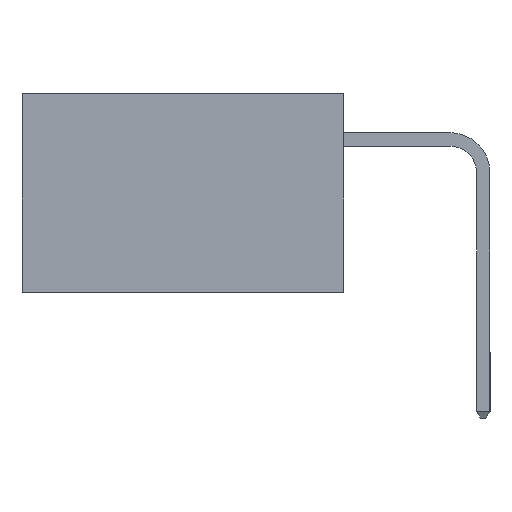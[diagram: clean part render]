
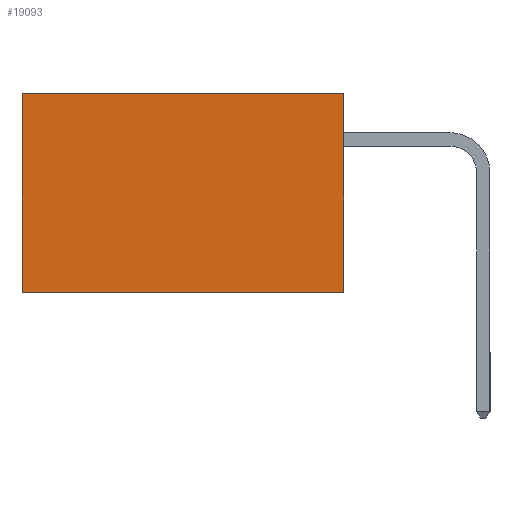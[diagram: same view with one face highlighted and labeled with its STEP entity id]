
A CAD part, left-side view. The second image highlights one B-rep face of the part: STEP entity #19093.
In plain terms, the highlighted planar face has unit normal (-1, 0, 0).
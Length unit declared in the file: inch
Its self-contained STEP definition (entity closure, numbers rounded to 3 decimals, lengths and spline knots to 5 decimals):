
#627 = DIRECTION ( 'NONE',  ( 0., 0., -1. ) ) ;
#920 = LINE ( 'NONE', #1211, #15203 ) ;
#930 = ORIENTED_EDGE ( 'NONE', *, *, #7329, .T. ) ;
#1211 = CARTESIAN_POINT ( 'NONE',  ( 0.2615, 0., 0. ) ) ;
#2139 = LINE ( 'NONE', #5293, #7869 ) ;
#2337 = CARTESIAN_POINT ( 'NONE',  ( 0.2615, 0., -0.37 ) ) ;
#5293 = CARTESIAN_POINT ( 'NONE',  ( 0.2615, 0.6, -0.37 ) ) ;
#5591 = VECTOR ( 'NONE', #17047, 39.37008 ) ;
#5892 = EDGE_CURVE ( 'NONE', #15554, #14529, #18136, .T. ) ;
#6039 = FACE_OUTER_BOUND ( 'NONE', #9363, .T. ) ;
#6125 = VERTEX_POINT ( 'NONE', #16425 ) ;
#7064 = VECTOR ( 'NONE', #15613, 39.37008 ) ;
#7329 = EDGE_CURVE ( 'NONE', #15351, #14529, #2139, .T. ) ;
#7866 = DIRECTION ( 'NONE',  ( 0., 0., -1. ) ) ;
#7869 = VECTOR ( 'NONE', #627, 39.37008 ) ;
#9349 = LINE ( 'NONE', #12423, #7064 ) ;
#9363 = EDGE_LOOP ( 'NONE', ( #930, #19481, #10016, #16071 ) ) ;
#9390 = PLANE ( 'NONE',  #11045 ) ;
#10016 = ORIENTED_EDGE ( 'NONE', *, *, #15057, .F. ) ;
#10208 = DIRECTION ( 'NONE',  ( 0., 1., 0. ) ) ;
#11045 = AXIS2_PLACEMENT_3D ( 'NONE', #13699, #15649, #7866 ) ;
#12305 = EDGE_CURVE ( 'NONE', #6125, #15351, #920, .T. ) ;
#12423 = CARTESIAN_POINT ( 'NONE',  ( 0.2615, 0., -0.37 ) ) ;
#13699 = CARTESIAN_POINT ( 'NONE',  ( 0.2615, 0., -0.37 ) ) ;
#14474 = CARTESIAN_POINT ( 'NONE',  ( 0.2615, 0.6, 0. ) ) ;
#14529 = VERTEX_POINT ( 'NONE', #14966 ) ;
#14966 = CARTESIAN_POINT ( 'NONE',  ( 0.2615, 0.6, -0.37 ) ) ;
#15057 = EDGE_CURVE ( 'NONE', #6125, #15554, #9349, .T. ) ;
#15203 = VECTOR ( 'NONE', #10208, 39.37008 ) ;
#15351 = VERTEX_POINT ( 'NONE', #14474 ) ;
#15554 = VERTEX_POINT ( 'NONE', #2337 ) ;
#15613 = DIRECTION ( 'NONE',  ( 0., 0., -1. ) ) ;
#15649 = DIRECTION ( 'NONE',  ( 1., 0., 0. ) ) ;
#16071 = ORIENTED_EDGE ( 'NONE', *, *, #12305, .T. ) ;
#16425 = CARTESIAN_POINT ( 'NONE',  ( 0.2615, 0., 0. ) ) ;
#17047 = DIRECTION ( 'NONE',  ( 0., 1., 0. ) ) ;
#18136 = LINE ( 'NONE', #19695, #5591 ) ;
#19093 = ADVANCED_FACE ( 'NONE', ( #6039 ), #9390, .F. ) ;
#19481 = ORIENTED_EDGE ( 'NONE', *, *, #5892, .F. ) ;
#19695 = CARTESIAN_POINT ( 'NONE',  ( 0.2615, 0., -0.37 ) ) ;
